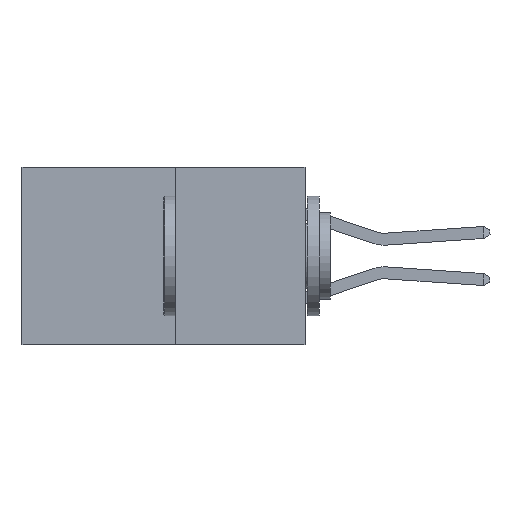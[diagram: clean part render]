
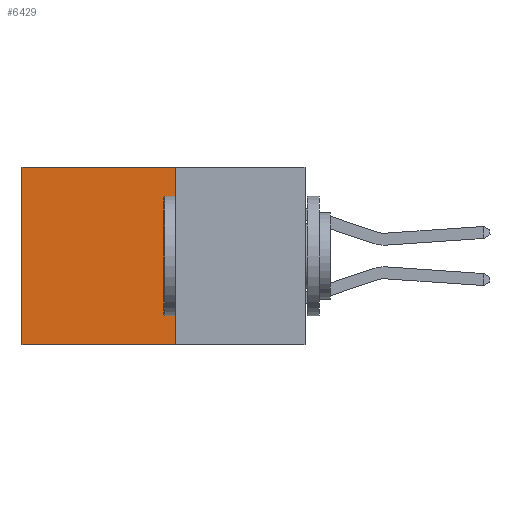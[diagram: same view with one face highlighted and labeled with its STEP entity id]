
A CAD part, left-side view. The second image highlights one B-rep face of the part: STEP entity #6429.
In plain terms, the highlighted planar face has unit normal (-1, 0, 0).
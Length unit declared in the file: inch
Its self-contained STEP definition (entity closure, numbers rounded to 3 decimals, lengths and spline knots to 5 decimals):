
#76 = VECTOR ( 'NONE', #7066, 39.37008 ) ;
#139 = ORIENTED_EDGE ( 'NONE', *, *, #1208, .T. ) ;
#197 = DIRECTION ( 'NONE',  ( 1., 0., 0. ) ) ;
#339 = PLANE ( 'NONE',  #7753 ) ;
#549 = CARTESIAN_POINT ( 'NONE',  ( 0.277, 0.27, -0.37 ) ) ;
#754 = EDGE_CURVE ( 'NONE', #1438, #4578, #1672, .T. ) ;
#904 = VERTEX_POINT ( 'NONE', #5130 ) ;
#976 = CARTESIAN_POINT ( 'NONE',  ( 0.277, 0.59, -0.37 ) ) ;
#980 = DIRECTION ( 'NONE',  ( 0., 1., 0. ) ) ;
#1208 = EDGE_CURVE ( 'NONE', #2218, #904, #3626, .T. ) ;
#1429 = EDGE_LOOP ( 'NONE', ( #2438, #1889, #1815, #139 ) ) ;
#1438 = VERTEX_POINT ( 'NONE', #5230 ) ;
#1455 = VECTOR ( 'NONE', #7121, 39.37008 ) ;
#1672 = LINE ( 'NONE', #6810, #1455 ) ;
#1815 = ORIENTED_EDGE ( 'NONE', *, *, #4817, .F. ) ;
#1889 = ORIENTED_EDGE ( 'NONE', *, *, #754, .F. ) ;
#2126 = CARTESIAN_POINT ( 'NONE',  ( 0.277, 0.27, 0. ) ) ;
#2218 = VERTEX_POINT ( 'NONE', #2126 ) ;
#2438 = ORIENTED_EDGE ( 'NONE', *, *, #3366, .T. ) ;
#3366 = EDGE_CURVE ( 'NONE', #904, #4578, #3857, .T. ) ;
#3626 = LINE ( 'NONE', #5318, #6663 ) ;
#3857 = LINE ( 'NONE', #7184, #76 ) ;
#4578 = VERTEX_POINT ( 'NONE', #976 ) ;
#4817 = EDGE_CURVE ( 'NONE', #2218, #1438, #8460, .T. ) ;
#5130 = CARTESIAN_POINT ( 'NONE',  ( 0.277, 0.59, 0. ) ) ;
#5230 = CARTESIAN_POINT ( 'NONE',  ( 0.277, 0.27, -0.37 ) ) ;
#5318 = CARTESIAN_POINT ( 'NONE',  ( 0.277, 0.27, 0. ) ) ;
#5363 = DIRECTION ( 'NONE',  ( 0., 0., -1. ) ) ;
#5391 = CARTESIAN_POINT ( 'NONE',  ( 0.277, 0.27, -0.37 ) ) ;
#6429 = ADVANCED_FACE ( 'NONE', ( #6844 ), #339, .F. ) ;
#6663 = VECTOR ( 'NONE', #980, 39.37008 ) ;
#6810 = CARTESIAN_POINT ( 'NONE',  ( 0.277, 0.27, -0.37 ) ) ;
#6844 = FACE_OUTER_BOUND ( 'NONE', #1429, .T. ) ;
#6966 = VECTOR ( 'NONE', #5363, 39.37008 ) ;
#7066 = DIRECTION ( 'NONE',  ( 0., 0., -1. ) ) ;
#7121 = DIRECTION ( 'NONE',  ( 0., 1., 0. ) ) ;
#7184 = CARTESIAN_POINT ( 'NONE',  ( 0.277, 0.59, -0.37 ) ) ;
#7753 = AXIS2_PLACEMENT_3D ( 'NONE', #549, #197, #8266 ) ;
#8266 = DIRECTION ( 'NONE',  ( 0., 0., -1. ) ) ;
#8460 = LINE ( 'NONE', #5391, #6966 ) ;
